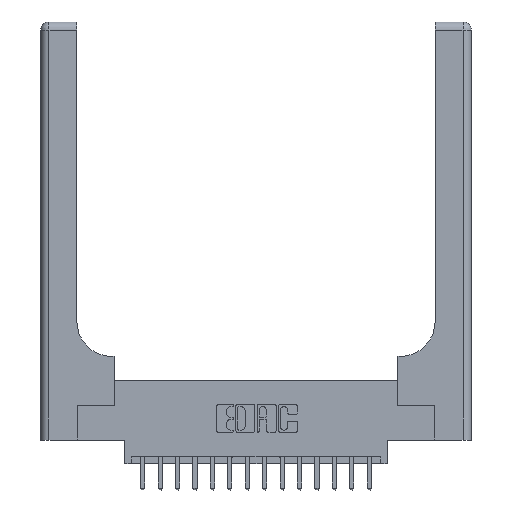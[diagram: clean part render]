
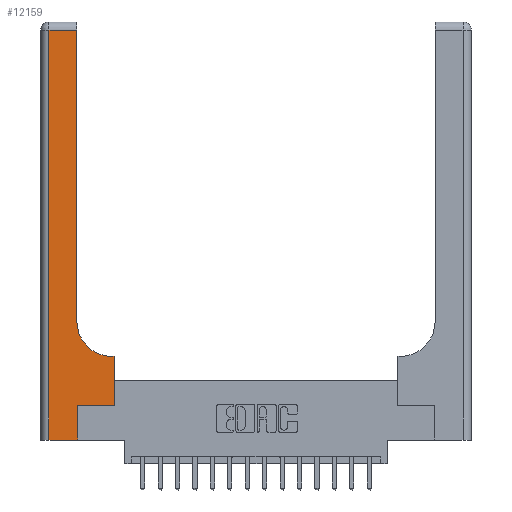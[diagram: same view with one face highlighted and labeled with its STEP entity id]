
A CAD part, top view. The second image highlights one B-rep face of the part: STEP entity #12159.
In plain terms, the highlighted planar face has unit normal (0, 0, 1).
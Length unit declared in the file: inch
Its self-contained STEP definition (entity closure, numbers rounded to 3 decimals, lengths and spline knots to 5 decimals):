
#589 = CARTESIAN_POINT ( 'NONE',  ( 0., 2.94, 0.37 ) ) ;
#909 = CARTESIAN_POINT ( 'NONE',  ( 0.51, 0.6, 0.37 ) ) ;
#990 = EDGE_LOOP ( 'NONE', ( #2887, #4768, #2759, #17147, #4690, #4416, #15362, #3749, #7719 ) ) ;
#1129 = LINE ( 'NONE', #8253, #3700 ) ;
#1573 = VERTEX_POINT ( 'NONE', #18299 ) ;
#1578 = VERTEX_POINT ( 'NONE', #9721 ) ;
#1723 = VECTOR ( 'NONE', #8745, 39.37008 ) ;
#2111 = DIRECTION ( 'NONE',  ( 0., 0., -1. ) ) ;
#2358 = VERTEX_POINT ( 'NONE', #11651 ) ;
#2759 = ORIENTED_EDGE ( 'NONE', *, *, #14722, .T. ) ;
#2887 = ORIENTED_EDGE ( 'NONE', *, *, #13562, .T. ) ;
#2944 = CARTESIAN_POINT ( 'NONE',  ( 0., 0., 0.37 ) ) ;
#3155 = PLANE ( 'NONE',  #10064 ) ;
#3700 = VECTOR ( 'NONE', #6806, 39.37008 ) ;
#3749 = ORIENTED_EDGE ( 'NONE', *, *, #13878, .T. ) ;
#4105 = EDGE_CURVE ( 'NONE', #1578, #4607, #14764, .T. ) ;
#4191 = LINE ( 'NONE', #2944, #1723 ) ;
#4416 = ORIENTED_EDGE ( 'NONE', *, *, #4105, .T. ) ;
#4607 = VERTEX_POINT ( 'NONE', #11010 ) ;
#4690 = ORIENTED_EDGE ( 'NONE', *, *, #18307, .T. ) ;
#4768 = ORIENTED_EDGE ( 'NONE', *, *, #8478, .T. ) ;
#5015 = LINE ( 'NONE', #589, #11474 ) ;
#5035 = CARTESIAN_POINT ( 'NONE',  ( 0.528, 0.25, 0.37 ) ) ;
#5564 = LINE ( 'NONE', #11362, #14749 ) ;
#5784 = VECTOR ( 'NONE', #13425, 39.37008 ) ;
#5971 = CARTESIAN_POINT ( 'NONE',  ( 0.26, 3., 0.37 ) ) ;
#6288 = CARTESIAN_POINT ( 'NONE',  ( 0.06, 2.94, 0.37 ) ) ;
#6521 = CARTESIAN_POINT ( 'NONE',  ( 0.265, 0., 0.37 ) ) ;
#6806 = DIRECTION ( 'NONE',  ( 0., -1., 0. ) ) ;
#7044 = DIRECTION ( 'NONE',  ( -1., 0., 0. ) ) ;
#7181 = EDGE_CURVE ( 'NONE', #2358, #8842, #4191, .T. ) ;
#7317 = AXIS2_PLACEMENT_3D ( 'NONE', #14901, #13462, #7982 ) ;
#7719 = ORIENTED_EDGE ( 'NONE', *, *, #14621, .T. ) ;
#7982 = DIRECTION ( 'NONE',  ( 1., 0., 0. ) ) ;
#8150 = EDGE_CURVE ( 'NONE', #4607, #1573, #18082, .T. ) ;
#8239 = VECTOR ( 'NONE', #7044, 39.37008 ) ;
#8253 = CARTESIAN_POINT ( 'NONE',  ( 0.06, 3., 0.37 ) ) ;
#8478 = EDGE_CURVE ( 'NONE', #13822, #13752, #5015, .T. ) ;
#8745 = DIRECTION ( 'NONE',  ( 1., 0., 0. ) ) ;
#8842 = VERTEX_POINT ( 'NONE', #6521 ) ;
#9620 = LINE ( 'NONE', #15417, #8239 ) ;
#9721 = CARTESIAN_POINT ( 'NONE',  ( 0.265, 0.25, 0.37 ) ) ;
#9789 = VERTEX_POINT ( 'NONE', #17967 ) ;
#10064 = AXIS2_PLACEMENT_3D ( 'NONE', #13601, #2111, #16274 ) ;
#10470 = FACE_OUTER_BOUND ( 'NONE', #990, .T. ) ;
#10820 = DIRECTION ( 'NONE',  ( -1., 0., 0. ) ) ;
#11010 = CARTESIAN_POINT ( 'NONE',  ( 0.528, 0.25, 0.37 ) ) ;
#11362 = CARTESIAN_POINT ( 'NONE',  ( 0.265, 0., 0.37 ) ) ;
#11474 = VECTOR ( 'NONE', #10820, 39.37008 ) ;
#11651 = CARTESIAN_POINT ( 'NONE',  ( 0.06, 0., 0.37 ) ) ;
#11718 = CARTESIAN_POINT ( 'NONE',  ( 0.265, 0.25, 0.37 ) ) ;
#11862 = DIRECTION ( 'NONE',  ( 0., 1., 0. ) ) ;
#12159 = ADVANCED_FACE ( 'NONE', ( #10470 ), #3155, .F. ) ;
#13425 = DIRECTION ( 'NONE',  ( 1., 0., 0. ) ) ;
#13462 = DIRECTION ( 'NONE',  ( 0., 0., -1. ) ) ;
#13562 = EDGE_CURVE ( 'NONE', #9789, #13822, #16157, .T. ) ;
#13601 = CARTESIAN_POINT ( 'NONE',  ( 0., 3., 0.37 ) ) ;
#13752 = VERTEX_POINT ( 'NONE', #6288 ) ;
#13822 = VERTEX_POINT ( 'NONE', #18581 ) ;
#13878 = EDGE_CURVE ( 'NONE', #1573, #16463, #9620, .T. ) ;
#14497 = VECTOR ( 'NONE', #16475, 39.37008 ) ;
#14621 = EDGE_CURVE ( 'NONE', #16463, #9789, #15530, .T. ) ;
#14722 = EDGE_CURVE ( 'NONE', #13752, #2358, #1129, .T. ) ;
#14749 = VECTOR ( 'NONE', #16106, 39.37008 ) ;
#14764 = LINE ( 'NONE', #11718, #5784 ) ;
#14901 = CARTESIAN_POINT ( 'NONE',  ( 0.51, 0.85, 0.37 ) ) ;
#15362 = ORIENTED_EDGE ( 'NONE', *, *, #8150, .T. ) ;
#15417 = CARTESIAN_POINT ( 'NONE',  ( 0.26, 0.6, 0.37 ) ) ;
#15530 = CIRCLE ( 'NONE', #7317, 0.25 ) ;
#16106 = DIRECTION ( 'NONE',  ( 0., 1., 0. ) ) ;
#16157 = LINE ( 'NONE', #5971, #17383 ) ;
#16274 = DIRECTION ( 'NONE',  ( -1., 0., 0. ) ) ;
#16463 = VERTEX_POINT ( 'NONE', #909 ) ;
#16475 = DIRECTION ( 'NONE',  ( 0., 1., 0. ) ) ;
#17147 = ORIENTED_EDGE ( 'NONE', *, *, #7181, .T. ) ;
#17383 = VECTOR ( 'NONE', #11862, 39.37008 ) ;
#17967 = CARTESIAN_POINT ( 'NONE',  ( 0.26, 0.85, 0.37 ) ) ;
#18082 = LINE ( 'NONE', #5035, #14497 ) ;
#18299 = CARTESIAN_POINT ( 'NONE',  ( 0.528, 0.6, 0.37 ) ) ;
#18307 = EDGE_CURVE ( 'NONE', #8842, #1578, #5564, .T. ) ;
#18581 = CARTESIAN_POINT ( 'NONE',  ( 0.26, 2.94, 0.37 ) ) ;
